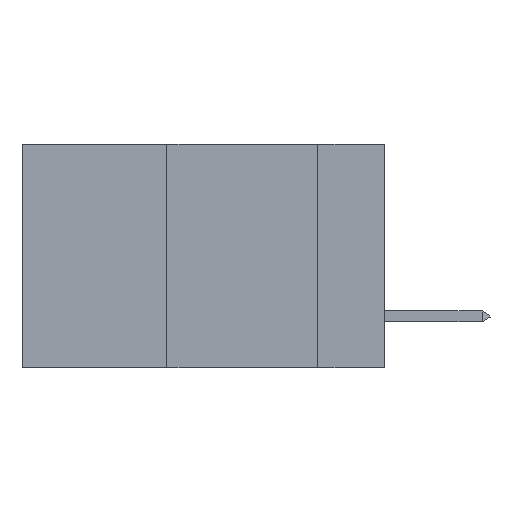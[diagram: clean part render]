
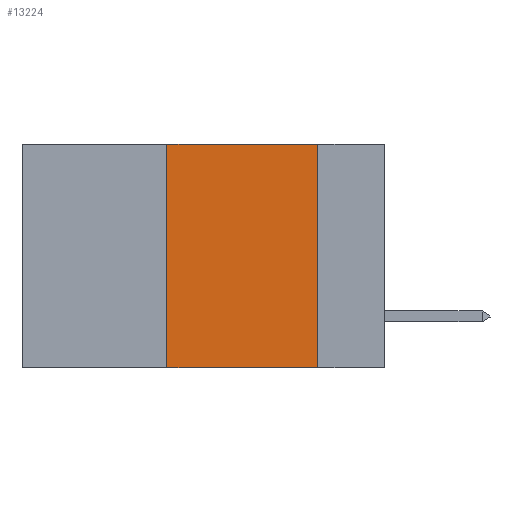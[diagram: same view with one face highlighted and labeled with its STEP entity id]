
A CAD part, left-side view. The second image highlights one B-rep face of the part: STEP entity #13224.
In plain terms, the highlighted planar face has unit normal (-1, 0, 0).
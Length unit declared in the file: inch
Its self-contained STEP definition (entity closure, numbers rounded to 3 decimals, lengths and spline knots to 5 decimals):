
#1841 = EDGE_CURVE ( 'NONE', #11430, #4514, #8265, .T. ) ;
#2682 = DIRECTION ( 'NONE',  ( 0., -1., 0. ) ) ;
#3652 = ORIENTED_EDGE ( 'NONE', *, *, #19737, .F. ) ;
#4514 = VERTEX_POINT ( 'NONE', #6133 ) ;
#5142 = VECTOR ( 'NONE', #16709, 39.37008 ) ;
#6133 = CARTESIAN_POINT ( 'NONE',  ( 0., 0.36, 0. ) ) ;
#6273 = CARTESIAN_POINT ( 'NONE',  ( 0., 0.11, 0. ) ) ;
#6405 = LINE ( 'NONE', #12606, #8357 ) ;
#7099 = DIRECTION ( 'NONE',  ( 0., 0., -1. ) ) ;
#8265 = LINE ( 'NONE', #13044, #25699 ) ;
#8357 = VECTOR ( 'NONE', #2682, 39.37008 ) ;
#8633 = FACE_OUTER_BOUND ( 'NONE', #24327, .T. ) ;
#9977 = VERTEX_POINT ( 'NONE', #21472 ) ;
#10314 = DIRECTION ( 'NONE',  ( 0., 0., -1. ) ) ;
#11430 = VERTEX_POINT ( 'NONE', #24362 ) ;
#11735 = ORIENTED_EDGE ( 'NONE', *, *, #17494, .F. ) ;
#12606 = CARTESIAN_POINT ( 'NONE',  ( 0., 0.6, 0. ) ) ;
#13044 = CARTESIAN_POINT ( 'NONE',  ( 0., 0.36, 0. ) ) ;
#13193 = DIRECTION ( 'NONE',  ( 1., 0., 0. ) ) ;
#13224 = ADVANCED_FACE ( 'NONE', ( #8633 ), #25305, .F. ) ;
#14005 = VECTOR ( 'NONE', #10314, 39.37008 ) ;
#14517 = ORIENTED_EDGE ( 'NONE', *, *, #1841, .F. ) ;
#15957 = LINE ( 'NONE', #16439, #5142 ) ;
#16439 = CARTESIAN_POINT ( 'NONE',  ( 0., 0.6, -0.37 ) ) ;
#16709 = DIRECTION ( 'NONE',  ( 0., -1., 0. ) ) ;
#16885 = ORIENTED_EDGE ( 'NONE', *, *, #18424, .T. ) ;
#17080 = DIRECTION ( 'NONE',  ( 0., 0., 1. ) ) ;
#17478 = VERTEX_POINT ( 'NONE', #22670 ) ;
#17494 = EDGE_CURVE ( 'NONE', #4514, #9977, #6405, .T. ) ;
#17596 = CARTESIAN_POINT ( 'NONE',  ( 0., 0.6, 0. ) ) ;
#18424 = EDGE_CURVE ( 'NONE', #11430, #17478, #15957, .T. ) ;
#19114 = AXIS2_PLACEMENT_3D ( 'NONE', #17596, #13193, #7099 ) ;
#19737 = EDGE_CURVE ( 'NONE', #9977, #17478, #20014, .T. ) ;
#20014 = LINE ( 'NONE', #6273, #14005 ) ;
#21472 = CARTESIAN_POINT ( 'NONE',  ( 0., 0.11, 0. ) ) ;
#22670 = CARTESIAN_POINT ( 'NONE',  ( 0., 0.11, -0.37 ) ) ;
#24327 = EDGE_LOOP ( 'NONE', ( #3652, #11735, #14517, #16885 ) ) ;
#24362 = CARTESIAN_POINT ( 'NONE',  ( 0., 0.36, -0.37 ) ) ;
#25305 = PLANE ( 'NONE',  #19114 ) ;
#25699 = VECTOR ( 'NONE', #17080, 39.37008 ) ;
